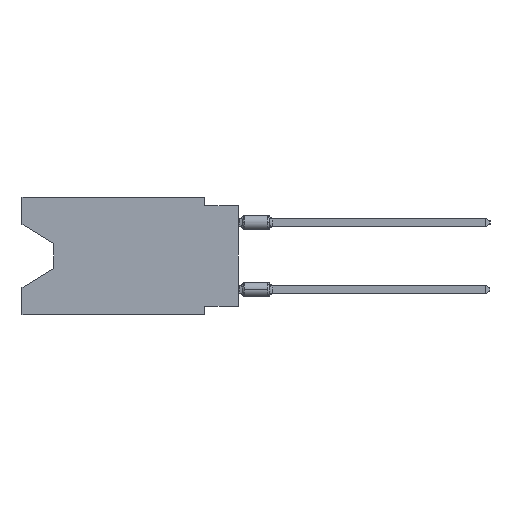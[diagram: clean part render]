
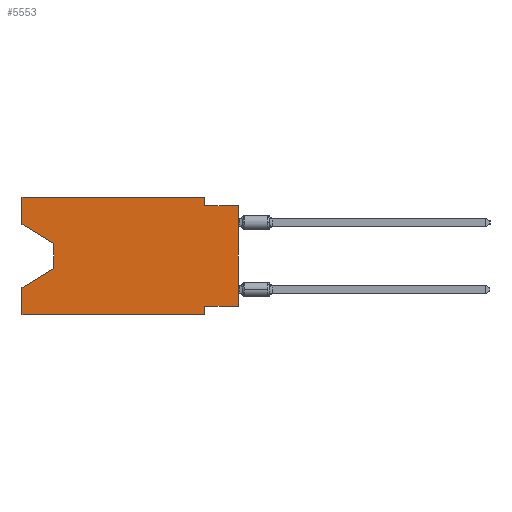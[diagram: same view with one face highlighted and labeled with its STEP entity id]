
A CAD part, left-side view. The second image highlights one B-rep face of the part: STEP entity #5553.
In plain terms, the highlighted planar face has unit normal (-1, 0, 0).
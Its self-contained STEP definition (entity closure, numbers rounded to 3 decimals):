
#405 = CARTESIAN_POINT ( 'NONE',  ( 0., 2.54, 0. ) ) ;
#611 = LINE ( 'NONE', #34601, #26104 ) ;
#980 = VERTEX_POINT ( 'NONE', #11487 ) ;
#1795 = CARTESIAN_POINT ( 'NONE',  ( 0., 13.97, -5.385 ) ) ;
#2036 = EDGE_CURVE ( 'NONE', #5527, #25293, #16734, .T. ) ;
#2141 = ORIENTED_EDGE ( 'NONE', *, *, #9191, .T. ) ;
#2513 = CARTESIAN_POINT ( 'NONE',  ( 0., 13.97, -3.505 ) ) ;
#2640 = AXIS2_PLACEMENT_3D ( 'NONE', #26909, #24471, #15405 ) ;
#3078 = ORIENTED_EDGE ( 'NONE', *, *, #17145, .F. ) ;
#3462 = VERTEX_POINT ( 'NONE', #405 ) ;
#3836 = CARTESIAN_POINT ( 'NONE',  ( 0., 16.383, 0. ) ) ;
#4066 = PLANE ( 'NONE',  #2640 ) ;
#4871 = DIRECTION ( 'NONE',  ( 0., 0., 1. ) ) ;
#5282 = VERTEX_POINT ( 'NONE', #17997 ) ;
#5477 = DIRECTION ( 'NONE',  ( 0., 0., -1. ) ) ;
#5527 = VERTEX_POINT ( 'NONE', #13143 ) ;
#5553 = ADVANCED_FACE ( 'NONE', ( #9793 ), #4066, .F. ) ;
#5942 = CARTESIAN_POINT ( 'NONE',  ( 0., 2.54, -8.89 ) ) ;
#6062 = DIRECTION ( 'NONE',  ( 0., -1., 0. ) ) ;
#7107 = VERTEX_POINT ( 'NONE', #9014 ) ;
#7314 = VECTOR ( 'NONE', #11379, 1000. ) ;
#7442 = DIRECTION ( 'NONE',  ( 0., 0., 1. ) ) ;
#8133 = CARTESIAN_POINT ( 'NONE',  ( 0., 2.54, 0. ) ) ;
#8654 = LINE ( 'NONE', #3836, #17279 ) ;
#9014 = CARTESIAN_POINT ( 'NONE',  ( 0., 16.383, -8.89 ) ) ;
#9113 = DIRECTION ( 'NONE',  ( 0., -1., 0. ) ) ;
#9150 = DIRECTION ( 'NONE',  ( 0., 1., 0. ) ) ;
#9191 = EDGE_CURVE ( 'NONE', #7107, #36377, #611, .T. ) ;
#9793 = FACE_OUTER_BOUND ( 'NONE', #18121, .T. ) ;
#10252 = VECTOR ( 'NONE', #5477, 1000. ) ;
#10443 = CARTESIAN_POINT ( 'NONE',  ( 0., 0., 0. ) ) ;
#10812 = VERTEX_POINT ( 'NONE', #24608 ) ;
#11379 = DIRECTION ( 'NONE',  ( 0., 0.855, -0.519 ) ) ;
#11418 = CARTESIAN_POINT ( 'NONE',  ( 0., 16.383, 0. ) ) ;
#11487 = CARTESIAN_POINT ( 'NONE',  ( 0., 2.54, -8.255 ) ) ;
#11811 = EDGE_CURVE ( 'NONE', #25293, #3462, #8654, .T. ) ;
#12547 = LINE ( 'NONE', #32420, #32807 ) ;
#12900 = VECTOR ( 'NONE', #35877, 1000. ) ;
#13143 = CARTESIAN_POINT ( 'NONE',  ( 0., 16.383, -2.038 ) ) ;
#13427 = LINE ( 'NONE', #10443, #14644 ) ;
#13594 = CARTESIAN_POINT ( 'NONE',  ( 0., 16.383, 0. ) ) ;
#13755 = CARTESIAN_POINT ( 'NONE',  ( 0., 16.383, 0. ) ) ;
#14000 = CARTESIAN_POINT ( 'NONE',  ( 0., 13.97, -5.385 ) ) ;
#14344 = ORIENTED_EDGE ( 'NONE', *, *, #28630, .F. ) ;
#14390 = CARTESIAN_POINT ( 'NONE',  ( 0., 0., -0.635 ) ) ;
#14644 = VECTOR ( 'NONE', #4871, 1000. ) ;
#14915 = EDGE_CURVE ( 'NONE', #3462, #5282, #18769, .T. ) ;
#15119 = CARTESIAN_POINT ( 'NONE',  ( 0., 0., -8.255 ) ) ;
#15192 = VECTOR ( 'NONE', #28606, 1000. ) ;
#15405 = DIRECTION ( 'NONE',  ( 0., 0., -1. ) ) ;
#15528 = DIRECTION ( 'NONE',  ( 0., -1., 0. ) ) ;
#15554 = EDGE_CURVE ( 'NONE', #5282, #17845, #12547, .T. ) ;
#15798 = EDGE_CURVE ( 'NONE', #23450, #16290, #17342, .T. ) ;
#16290 = VERTEX_POINT ( 'NONE', #29683 ) ;
#16734 = LINE ( 'NONE', #13594, #12900 ) ;
#17145 = EDGE_CURVE ( 'NONE', #7107, #16290, #27894, .T. ) ;
#17279 = VECTOR ( 'NONE', #6062, 1000. ) ;
#17342 = LINE ( 'NONE', #14000, #7314 ) ;
#17459 = CARTESIAN_POINT ( 'NONE',  ( 0., 2.54, -8.89 ) ) ;
#17845 = VERTEX_POINT ( 'NONE', #14390 ) ;
#17997 = CARTESIAN_POINT ( 'NONE',  ( 0., 2.54, -0.635 ) ) ;
#18121 = EDGE_LOOP ( 'NONE', ( #35508, #19054, #20677, #3078, #2141, #25904, #14344, #30197, #33448, #23677, #32611, #23682 ) ) ;
#18769 = LINE ( 'NONE', #8133, #35139 ) ;
#18797 = LINE ( 'NONE', #30467, #30793 ) ;
#18960 = EDGE_CURVE ( 'NONE', #25715, #23450, #33196, .T. ) ;
#19054 = ORIENTED_EDGE ( 'NONE', *, *, #18960, .T. ) ;
#20677 = ORIENTED_EDGE ( 'NONE', *, *, #15798, .T. ) ;
#21220 = DIRECTION ( 'NONE',  ( 0., -0.855, -0.519 ) ) ;
#23450 = VERTEX_POINT ( 'NONE', #1795 ) ;
#23677 = ORIENTED_EDGE ( 'NONE', *, *, #14915, .F. ) ;
#23682 = ORIENTED_EDGE ( 'NONE', *, *, #2036, .F. ) ;
#24471 = DIRECTION ( 'NONE',  ( 1., 0., 0. ) ) ;
#24608 = CARTESIAN_POINT ( 'NONE',  ( 0., 0., -8.255 ) ) ;
#25293 = VERTEX_POINT ( 'NONE', #11418 ) ;
#25715 = VERTEX_POINT ( 'NONE', #29220 ) ;
#25785 = VECTOR ( 'NONE', #7442, 1000. ) ;
#25904 = ORIENTED_EDGE ( 'NONE', *, *, #36416, .F. ) ;
#25909 = LINE ( 'NONE', #15119, #30770 ) ;
#26104 = VECTOR ( 'NONE', #9113, 1000. ) ;
#26909 = CARTESIAN_POINT ( 'NONE',  ( 0., 16.383, 0. ) ) ;
#27894 = LINE ( 'NONE', #13755, #25785 ) ;
#28606 = DIRECTION ( 'NONE',  ( 0., 0., -1. ) ) ;
#28630 = EDGE_CURVE ( 'NONE', #10812, #980, #25909, .T. ) ;
#29118 = EDGE_CURVE ( 'NONE', #5527, #25715, #18797, .T. ) ;
#29220 = CARTESIAN_POINT ( 'NONE',  ( 0., 13.97, -3.505 ) ) ;
#29683 = CARTESIAN_POINT ( 'NONE',  ( 0., 16.383, -6.852 ) ) ;
#30092 = DIRECTION ( 'NONE',  ( 0., 0., -1. ) ) ;
#30197 = ORIENTED_EDGE ( 'NONE', *, *, #34524, .T. ) ;
#30467 = CARTESIAN_POINT ( 'NONE',  ( 0., 16.383, -2.038 ) ) ;
#30770 = VECTOR ( 'NONE', #9150, 1000. ) ;
#30793 = VECTOR ( 'NONE', #21220, 1000. ) ;
#32420 = CARTESIAN_POINT ( 'NONE',  ( 0., 0., -0.635 ) ) ;
#32611 = ORIENTED_EDGE ( 'NONE', *, *, #11811, .F. ) ;
#32807 = VECTOR ( 'NONE', #15528, 1000. ) ;
#33196 = LINE ( 'NONE', #2513, #10252 ) ;
#33448 = ORIENTED_EDGE ( 'NONE', *, *, #15554, .F. ) ;
#34189 = LINE ( 'NONE', #5942, #15192 ) ;
#34524 = EDGE_CURVE ( 'NONE', #10812, #17845, #13427, .T. ) ;
#34601 = CARTESIAN_POINT ( 'NONE',  ( 0., 16.383, -8.89 ) ) ;
#35139 = VECTOR ( 'NONE', #30092, 1000. ) ;
#35508 = ORIENTED_EDGE ( 'NONE', *, *, #29118, .T. ) ;
#35877 = DIRECTION ( 'NONE',  ( 0., 0., 1. ) ) ;
#36377 = VERTEX_POINT ( 'NONE', #17459 ) ;
#36416 = EDGE_CURVE ( 'NONE', #980, #36377, #34189, .T. ) ;
